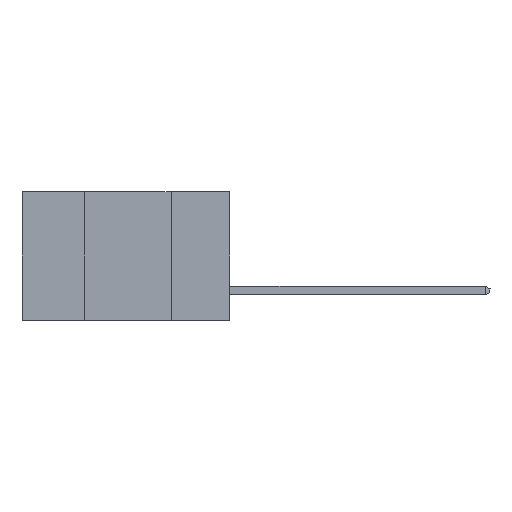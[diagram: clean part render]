
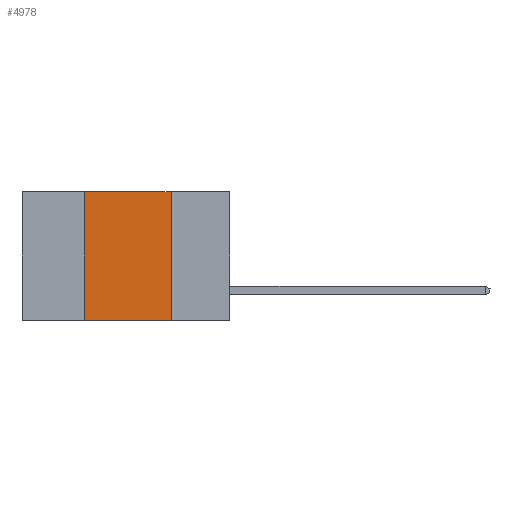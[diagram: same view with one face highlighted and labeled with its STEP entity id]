
A CAD part, left-side view. The second image highlights one B-rep face of the part: STEP entity #4978.
In plain terms, the highlighted planar face has unit normal (-1, 0, 0).
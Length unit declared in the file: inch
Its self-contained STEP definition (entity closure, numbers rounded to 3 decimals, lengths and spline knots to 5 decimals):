
#167 = ORIENTED_EDGE ( 'NONE', *, *, #6546, .F. ) ;
#244 = LINE ( 'NONE', #4949, #5335 ) ;
#278 = EDGE_CURVE ( 'NONE', #1087, #2263, #244, .T. ) ;
#467 = EDGE_CURVE ( 'NONE', #3502, #5815, #1128, .T. ) ;
#760 = LINE ( 'NONE', #2276, #2595 ) ;
#781 = CARTESIAN_POINT ( 'NONE',  ( 0., 0.17, 0. ) ) ;
#786 = EDGE_CURVE ( 'NONE', #3502, #2263, #760, .T. ) ;
#952 = DIRECTION ( 'NONE',  ( 0., 0., -1. ) ) ;
#1087 = VERTEX_POINT ( 'NONE', #781 ) ;
#1121 = EDGE_LOOP ( 'NONE', ( #2944, #167, #5865, #4836 ) ) ;
#1128 = LINE ( 'NONE', #7958, #1729 ) ;
#1515 = DIRECTION ( 'NONE',  ( 0., -1., 0. ) ) ;
#1729 = VECTOR ( 'NONE', #5211, 39.37008 ) ;
#2263 = VERTEX_POINT ( 'NONE', #2983 ) ;
#2276 = CARTESIAN_POINT ( 'NONE',  ( 0., 0.6, -0.37 ) ) ;
#2595 = VECTOR ( 'NONE', #1515, 39.37008 ) ;
#2944 = ORIENTED_EDGE ( 'NONE', *, *, #278, .F. ) ;
#2983 = CARTESIAN_POINT ( 'NONE',  ( 0., 0.17, -0.37 ) ) ;
#3500 = LINE ( 'NONE', #7453, #6906 ) ;
#3502 = VERTEX_POINT ( 'NONE', #4891 ) ;
#3776 = DIRECTION ( 'NONE',  ( 0., 0., -1. ) ) ;
#4082 = DIRECTION ( 'NONE',  ( 0., -1., 0. ) ) ;
#4836 = ORIENTED_EDGE ( 'NONE', *, *, #786, .T. ) ;
#4863 = CARTESIAN_POINT ( 'NONE',  ( 0., 0.42, 0. ) ) ;
#4891 = CARTESIAN_POINT ( 'NONE',  ( 0., 0.42, -0.37 ) ) ;
#4949 = CARTESIAN_POINT ( 'NONE',  ( 0., 0.17, -0.37 ) ) ;
#4978 = ADVANCED_FACE ( 'NONE', ( #5111 ), #5899, .F. ) ;
#5111 = FACE_OUTER_BOUND ( 'NONE', #1121, .T. ) ;
#5211 = DIRECTION ( 'NONE',  ( 0., 0., 1. ) ) ;
#5335 = VECTOR ( 'NONE', #952, 39.37008 ) ;
#5815 = VERTEX_POINT ( 'NONE', #4863 ) ;
#5865 = ORIENTED_EDGE ( 'NONE', *, *, #467, .F. ) ;
#5899 = PLANE ( 'NONE',  #6306 ) ;
#5977 = DIRECTION ( 'NONE',  ( 1., 0., 0. ) ) ;
#6306 = AXIS2_PLACEMENT_3D ( 'NONE', #8612, #5977, #3776 ) ;
#6546 = EDGE_CURVE ( 'NONE', #5815, #1087, #3500, .T. ) ;
#6906 = VECTOR ( 'NONE', #4082, 39.37008 ) ;
#7453 = CARTESIAN_POINT ( 'NONE',  ( 0., 0.6, 0. ) ) ;
#7958 = CARTESIAN_POINT ( 'NONE',  ( 0., 0.42, -0.37 ) ) ;
#8612 = CARTESIAN_POINT ( 'NONE',  ( 0., 0.6, 0. ) ) ;
